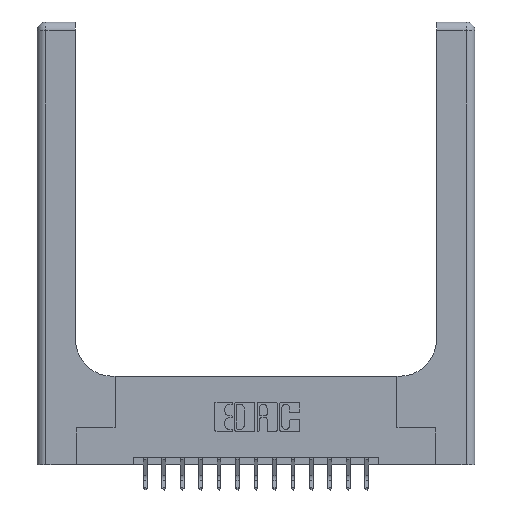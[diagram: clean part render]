
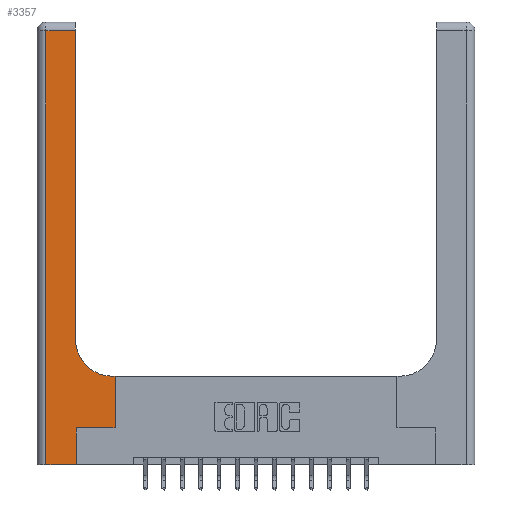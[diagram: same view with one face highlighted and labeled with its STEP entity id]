
A CAD part, top view. The second image highlights one B-rep face of the part: STEP entity #3357.
In plain terms, the highlighted planar face has unit normal (0, 0, 1).
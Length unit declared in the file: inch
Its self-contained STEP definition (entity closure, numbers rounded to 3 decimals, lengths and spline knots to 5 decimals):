
#1 = ORIENTED_EDGE ( 'NONE', *, *, #12270, .T. ) ;
#122 = CARTESIAN_POINT ( 'NONE',  ( 0.265, 0., 0.37 ) ) ;
#254 = VECTOR ( 'NONE', #16193, 39.37008 ) ;
#458 = DIRECTION ( 'NONE',  ( 0., 1., 0. ) ) ;
#638 = VERTEX_POINT ( 'NONE', #9242 ) ;
#736 = AXIS2_PLACEMENT_3D ( 'NONE', #12893, #1680, #4640 ) ;
#807 = VECTOR ( 'NONE', #458, 39.37008 ) ;
#1009 = EDGE_CURVE ( 'NONE', #7317, #638, #18121, .T. ) ;
#1064 = DIRECTION ( 'NONE',  ( -1., 0., 0. ) ) ;
#1121 = LINE ( 'NONE', #9852, #14624 ) ;
#1507 = EDGE_CURVE ( 'NONE', #16440, #5947, #5216, .T. ) ;
#1680 = DIRECTION ( 'NONE',  ( 0., 0., -1. ) ) ;
#1700 = DIRECTION ( 'NONE',  ( 0., 0., -1. ) ) ;
#1806 = ORIENTED_EDGE ( 'NONE', *, *, #11502, .T. ) ;
#1858 = LINE ( 'NONE', #11861, #254 ) ;
#2275 = VECTOR ( 'NONE', #1064, 39.37008 ) ;
#2307 = VERTEX_POINT ( 'NONE', #17680 ) ;
#3357 = ADVANCED_FACE ( 'NONE', ( #16114 ), #8919, .F. ) ;
#3604 = ORIENTED_EDGE ( 'NONE', *, *, #9361, .T. ) ;
#3829 = LINE ( 'NONE', #8170, #11476 ) ;
#4640 = DIRECTION ( 'NONE',  ( 1., 0., 0. ) ) ;
#4842 = ORIENTED_EDGE ( 'NONE', *, *, #15752, .T. ) ;
#5216 = LINE ( 'NONE', #16665, #2275 ) ;
#5255 = CARTESIAN_POINT ( 'NONE',  ( 0.06, 2.94, 0.37 ) ) ;
#5947 = VERTEX_POINT ( 'NONE', #5255 ) ;
#5960 = DIRECTION ( 'NONE',  ( -1., 0., 0. ) ) ;
#6053 = CARTESIAN_POINT ( 'NONE',  ( 0.51, 0.6, 0.37 ) ) ;
#6332 = CARTESIAN_POINT ( 'NONE',  ( 0.26, 3., 0.37 ) ) ;
#6428 = LINE ( 'NONE', #6332, #10601 ) ;
#6469 = ORIENTED_EDGE ( 'NONE', *, *, #14813, .T. ) ;
#6750 = DIRECTION ( 'NONE',  ( 0., -1., 0. ) ) ;
#7221 = ORIENTED_EDGE ( 'NONE', *, *, #1009, .T. ) ;
#7317 = VERTEX_POINT ( 'NONE', #14480 ) ;
#7402 = DIRECTION ( 'NONE',  ( -1., 0., 0. ) ) ;
#7697 = VERTEX_POINT ( 'NONE', #11029 ) ;
#7713 = DIRECTION ( 'NONE',  ( 0., 1., 0. ) ) ;
#7947 = ORIENTED_EDGE ( 'NONE', *, *, #17971, .T. ) ;
#8170 = CARTESIAN_POINT ( 'NONE',  ( 0., 0., 0.37 ) ) ;
#8919 = PLANE ( 'NONE',  #12075 ) ;
#9242 = CARTESIAN_POINT ( 'NONE',  ( 0.528, 0.6, 0.37 ) ) ;
#9361 = EDGE_CURVE ( 'NONE', #638, #11794, #12955, .T. ) ;
#9558 = ORIENTED_EDGE ( 'NONE', *, *, #17100, .T. ) ;
#9852 = CARTESIAN_POINT ( 'NONE',  ( 0.06, 3., 0.37 ) ) ;
#9861 = VECTOR ( 'NONE', #7402, 39.37008 ) ;
#9934 = CIRCLE ( 'NONE', #736, 0.25 ) ;
#9959 = LINE ( 'NONE', #122, #16853 ) ;
#10073 = CARTESIAN_POINT ( 'NONE',  ( 0.26, 0.85, 0.37 ) ) ;
#10601 = VECTOR ( 'NONE', #7713, 39.37008 ) ;
#10927 = VERTEX_POINT ( 'NONE', #11345 ) ;
#11029 = CARTESIAN_POINT ( 'NONE',  ( 0.265, 0.25, 0.37 ) ) ;
#11345 = CARTESIAN_POINT ( 'NONE',  ( 0.06, 0., 0.37 ) ) ;
#11476 = VECTOR ( 'NONE', #12535, 39.37008 ) ;
#11502 = EDGE_CURVE ( 'NONE', #15286, #16440, #6428, .T. ) ;
#11789 = CARTESIAN_POINT ( 'NONE',  ( 0., 3., 0.37 ) ) ;
#11794 = VERTEX_POINT ( 'NONE', #6053 ) ;
#11861 = CARTESIAN_POINT ( 'NONE',  ( 0.265, 0.25, 0.37 ) ) ;
#12075 = AXIS2_PLACEMENT_3D ( 'NONE', #11789, #1700, #5960 ) ;
#12270 = EDGE_CURVE ( 'NONE', #7697, #7317, #1858, .T. ) ;
#12535 = DIRECTION ( 'NONE',  ( 1., 0., 0. ) ) ;
#12893 = CARTESIAN_POINT ( 'NONE',  ( 0.51, 0.85, 0.37 ) ) ;
#12955 = LINE ( 'NONE', #17173, #9861 ) ;
#13198 = EDGE_LOOP ( 'NONE', ( #1806, #18159, #9558, #6469, #4842, #1, #7221, #3604, #7947 ) ) ;
#14480 = CARTESIAN_POINT ( 'NONE',  ( 0.528, 0.25, 0.37 ) ) ;
#14624 = VECTOR ( 'NONE', #6750, 39.37008 ) ;
#14813 = EDGE_CURVE ( 'NONE', #10927, #2307, #3829, .T. ) ;
#15286 = VERTEX_POINT ( 'NONE', #10073 ) ;
#15408 = CARTESIAN_POINT ( 'NONE',  ( 0.528, 0.25, 0.37 ) ) ;
#15748 = DIRECTION ( 'NONE',  ( 0., 1., 0. ) ) ;
#15752 = EDGE_CURVE ( 'NONE', #2307, #7697, #9959, .T. ) ;
#15765 = CARTESIAN_POINT ( 'NONE',  ( 0.26, 2.94, 0.37 ) ) ;
#16114 = FACE_OUTER_BOUND ( 'NONE', #13198, .T. ) ;
#16193 = DIRECTION ( 'NONE',  ( 1., 0., 0. ) ) ;
#16440 = VERTEX_POINT ( 'NONE', #15765 ) ;
#16665 = CARTESIAN_POINT ( 'NONE',  ( 0., 2.94, 0.37 ) ) ;
#16853 = VECTOR ( 'NONE', #15748, 39.37008 ) ;
#17100 = EDGE_CURVE ( 'NONE', #5947, #10927, #1121, .T. ) ;
#17173 = CARTESIAN_POINT ( 'NONE',  ( 0.26, 0.6, 0.37 ) ) ;
#17680 = CARTESIAN_POINT ( 'NONE',  ( 0.265, 0., 0.37 ) ) ;
#17971 = EDGE_CURVE ( 'NONE', #11794, #15286, #9934, .T. ) ;
#18121 = LINE ( 'NONE', #15408, #807 ) ;
#18159 = ORIENTED_EDGE ( 'NONE', *, *, #1507, .T. ) ;
